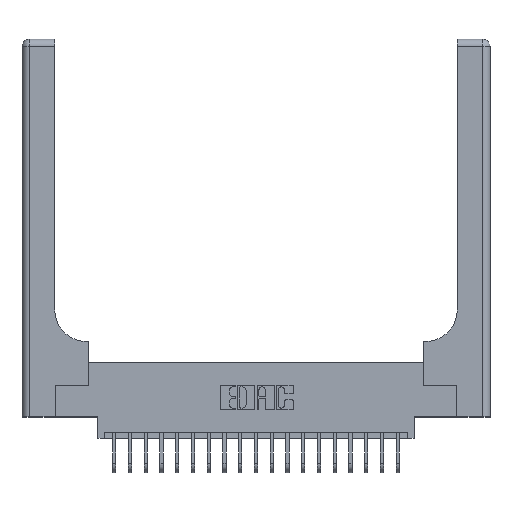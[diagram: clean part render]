
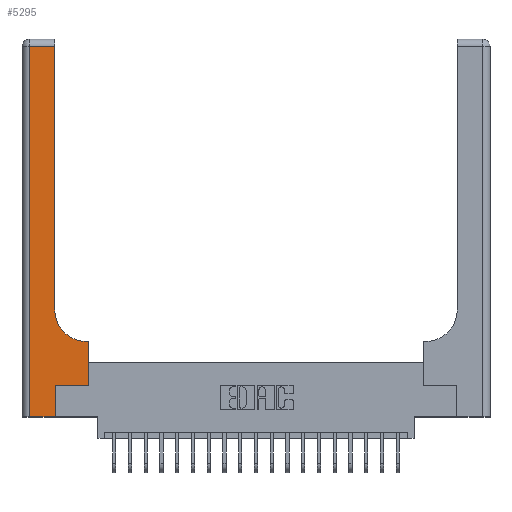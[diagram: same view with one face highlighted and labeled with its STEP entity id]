
A CAD part, top view. The second image highlights one B-rep face of the part: STEP entity #5295.
In plain terms, the highlighted planar face has unit normal (0, 0, 1).
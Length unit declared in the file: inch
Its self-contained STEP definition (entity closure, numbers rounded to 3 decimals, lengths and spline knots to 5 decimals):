
#87 = VERTEX_POINT ( 'NONE', #22419 ) ;
#185 = ORIENTED_EDGE ( 'NONE', *, *, #2574, .T. ) ;
#773 = CARTESIAN_POINT ( 'NONE',  ( 0.26, 0.6, 0.37 ) ) ;
#850 = CARTESIAN_POINT ( 'NONE',  ( 0.528, 0.25, 0.37 ) ) ;
#913 = LINE ( 'NONE', #2893, #11159 ) ;
#924 = VECTOR ( 'NONE', #19051, 39.37008 ) ;
#999 = LINE ( 'NONE', #773, #5437 ) ;
#1244 = VERTEX_POINT ( 'NONE', #16595 ) ;
#1815 = DIRECTION ( 'NONE',  ( 1., 0., 0. ) ) ;
#2285 = EDGE_CURVE ( 'NONE', #10542, #87, #20232, .T. ) ;
#2574 = EDGE_CURVE ( 'NONE', #8596, #18292, #14165, .T. ) ;
#2893 = CARTESIAN_POINT ( 'NONE',  ( 0.26, 3., 0.37 ) ) ;
#3299 = CARTESIAN_POINT ( 'NONE',  ( 0.528, 0.25, 0.37 ) ) ;
#3552 = CARTESIAN_POINT ( 'NONE',  ( 0., 0., 0.37 ) ) ;
#3826 = VERTEX_POINT ( 'NONE', #850 ) ;
#3916 = EDGE_CURVE ( 'NONE', #3826, #12364, #8669, .T. ) ;
#5295 = ADVANCED_FACE ( 'NONE', ( #21947 ), #9129, .F. ) ;
#5437 = VECTOR ( 'NONE', #9764, 39.37008 ) ;
#5511 = DIRECTION ( 'NONE',  ( 0., 0., -1. ) ) ;
#5512 = CARTESIAN_POINT ( 'NONE',  ( 0.265, 0., 0.37 ) ) ;
#5631 = DIRECTION ( 'NONE',  ( -1., 0., 0. ) ) ;
#5869 = ORIENTED_EDGE ( 'NONE', *, *, #2285, .T. ) ;
#6596 = EDGE_CURVE ( 'NONE', #87, #8596, #19528, .T. ) ;
#6687 = LINE ( 'NONE', #11819, #10039 ) ;
#8404 = CARTESIAN_POINT ( 'NONE',  ( 0., 2.94, 0.37 ) ) ;
#8484 = EDGE_CURVE ( 'NONE', #12364, #1244, #999, .T. ) ;
#8596 = VERTEX_POINT ( 'NONE', #5512 ) ;
#8669 = LINE ( 'NONE', #3299, #924 ) ;
#8838 = AXIS2_PLACEMENT_3D ( 'NONE', #21250, #10533, #17537 ) ;
#9106 = VECTOR ( 'NONE', #12898, 39.37008 ) ;
#9129 = PLANE ( 'NONE',  #16195 ) ;
#9360 = CARTESIAN_POINT ( 'NONE',  ( 0., 3., 0.37 ) ) ;
#9667 = EDGE_CURVE ( 'NONE', #1244, #19879, #18531, .T. ) ;
#9764 = DIRECTION ( 'NONE',  ( -1., 0., 0. ) ) ;
#10039 = VECTOR ( 'NONE', #19048, 39.37008 ) ;
#10230 = VECTOR ( 'NONE', #1815, 39.37008 ) ;
#10389 = DIRECTION ( 'NONE',  ( -1., 0., 0. ) ) ;
#10533 = DIRECTION ( 'NONE',  ( 0., 0., -1. ) ) ;
#10542 = VERTEX_POINT ( 'NONE', #14842 ) ;
#10615 = ORIENTED_EDGE ( 'NONE', *, *, #8484, .T. ) ;
#11159 = VECTOR ( 'NONE', #16897, 39.37008 ) ;
#11500 = CARTESIAN_POINT ( 'NONE',  ( 0.26, 0.85, 0.37 ) ) ;
#11566 = VECTOR ( 'NONE', #10389, 39.37008 ) ;
#11819 = CARTESIAN_POINT ( 'NONE',  ( 0.265, 0.25, 0.37 ) ) ;
#12010 = EDGE_CURVE ( 'NONE', #18292, #3826, #6687, .T. ) ;
#12015 = ORIENTED_EDGE ( 'NONE', *, *, #9667, .T. ) ;
#12028 = ORIENTED_EDGE ( 'NONE', *, *, #3916, .T. ) ;
#12364 = VERTEX_POINT ( 'NONE', #22167 ) ;
#12375 = CARTESIAN_POINT ( 'NONE',  ( 0.26, 2.94, 0.37 ) ) ;
#12525 = DIRECTION ( 'NONE',  ( 0., 1., 0. ) ) ;
#12718 = ORIENTED_EDGE ( 'NONE', *, *, #12010, .T. ) ;
#12898 = DIRECTION ( 'NONE',  ( 0., -1., 0. ) ) ;
#14049 = CARTESIAN_POINT ( 'NONE',  ( 0.265, 0., 0.37 ) ) ;
#14065 = EDGE_CURVE ( 'NONE', #19879, #18099, #913, .T. ) ;
#14165 = LINE ( 'NONE', #14049, #15163 ) ;
#14302 = ORIENTED_EDGE ( 'NONE', *, *, #6596, .T. ) ;
#14842 = CARTESIAN_POINT ( 'NONE',  ( 0.06, 2.94, 0.37 ) ) ;
#15163 = VECTOR ( 'NONE', #12525, 39.37008 ) ;
#15431 = EDGE_CURVE ( 'NONE', #18099, #10542, #20874, .T. ) ;
#16195 = AXIS2_PLACEMENT_3D ( 'NONE', #9360, #5511, #5631 ) ;
#16595 = CARTESIAN_POINT ( 'NONE',  ( 0.51, 0.6, 0.37 ) ) ;
#16897 = DIRECTION ( 'NONE',  ( 0., 1., 0. ) ) ;
#17537 = DIRECTION ( 'NONE',  ( 1., 0., 0. ) ) ;
#18095 = ORIENTED_EDGE ( 'NONE', *, *, #14065, .T. ) ;
#18099 = VERTEX_POINT ( 'NONE', #12375 ) ;
#18292 = VERTEX_POINT ( 'NONE', #18663 ) ;
#18531 = CIRCLE ( 'NONE', #8838, 0.25 ) ;
#18663 = CARTESIAN_POINT ( 'NONE',  ( 0.265, 0.25, 0.37 ) ) ;
#18691 = EDGE_LOOP ( 'NONE', ( #18095, #19668, #5869, #14302, #185, #12718, #12028, #10615, #12015 ) ) ;
#19048 = DIRECTION ( 'NONE',  ( 1., 0., 0. ) ) ;
#19051 = DIRECTION ( 'NONE',  ( 0., 1., 0. ) ) ;
#19528 = LINE ( 'NONE', #3552, #10230 ) ;
#19668 = ORIENTED_EDGE ( 'NONE', *, *, #15431, .T. ) ;
#19879 = VERTEX_POINT ( 'NONE', #11500 ) ;
#20232 = LINE ( 'NONE', #21637, #9106 ) ;
#20874 = LINE ( 'NONE', #8404, #11566 ) ;
#21250 = CARTESIAN_POINT ( 'NONE',  ( 0.51, 0.85, 0.37 ) ) ;
#21637 = CARTESIAN_POINT ( 'NONE',  ( 0.06, 3., 0.37 ) ) ;
#21947 = FACE_OUTER_BOUND ( 'NONE', #18691, .T. ) ;
#22167 = CARTESIAN_POINT ( 'NONE',  ( 0.528, 0.6, 0.37 ) ) ;
#22419 = CARTESIAN_POINT ( 'NONE',  ( 0.06, 0., 0.37 ) ) ;
